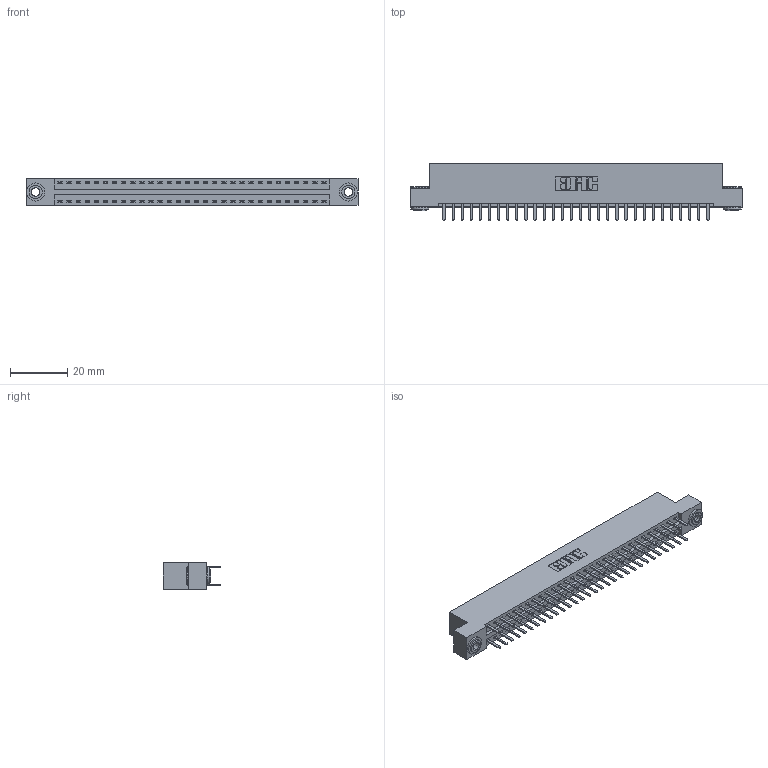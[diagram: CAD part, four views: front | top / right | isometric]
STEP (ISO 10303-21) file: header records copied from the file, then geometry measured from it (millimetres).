
FILE_DESCRIPTION (( 'STEP AP203' ), '1' );
FILE_NAME ('346-060-520-203.STEP', '2018-08-28T05:13:11', ( '' ), ( '' ), 'SwSTEP 2.0', 'SolidWorks 2016', '' );
FILE_SCHEMA (( 'CONFIG_CONTROL_DESIGN' ));
Length unit declared in the file: inch
Products named in the file (4): 346 Part_Flush Mounting Lugs - 0.156 Dia-TH; 345-292-001_345-293-120; 345-250-002_345-250-002-102; 346-060-520-203
Assembly tree (63 placements, depth 2):
  346-060-520-203
    346 Part_Flush Mounting Lugs - 0.156 Dia-TH
    345-292-001_345-293-120  x60
    345-250-002_345-250-002-102  x2
Bounding box: 115.82 x 20.02 x 9.4 mm (x, y, z)
Volume: 11194.1 mm3; surface area: 15350.8 mm2
Topology: 63 solids, 63 shells, 3520 faces, 10185 edges, 6626 vertices
Faces by surface type: plane 2306, cylinder 1206, cone 8
Entity records: 21958 total; most frequent: CARTESIAN_POINT 3623, ORIENTED_EDGE 3538, DIRECTION 3263, EDGE_CURVE 1769, VECTOR 1489, LINE 1489, VERTEX_POINT 1174, AXIS2_PLACEMENT_3D 887
